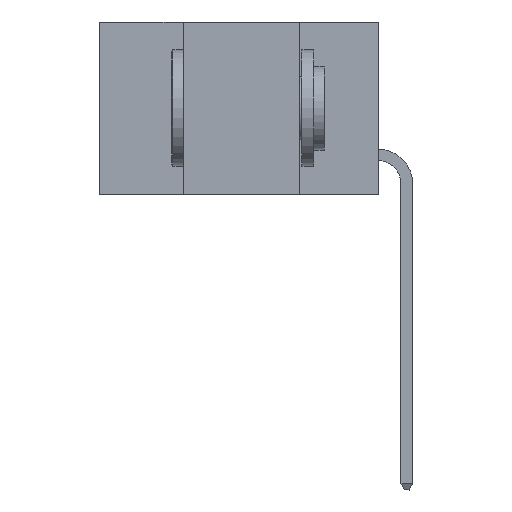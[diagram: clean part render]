
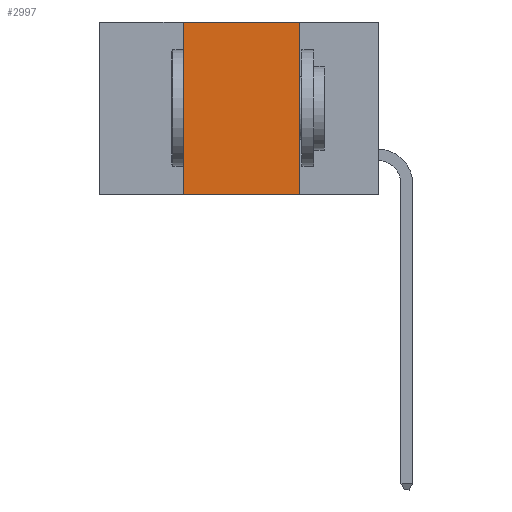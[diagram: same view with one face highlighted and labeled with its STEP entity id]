
A CAD part, left-side view. The second image highlights one B-rep face of the part: STEP entity #2997.
In plain terms, the highlighted planar face has unit normal (-1, 0, 0).
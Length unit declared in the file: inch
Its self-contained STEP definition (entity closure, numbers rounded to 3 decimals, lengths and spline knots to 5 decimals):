
#90 = ORIENTED_EDGE ( 'NONE', *, *, #4357, .F. ) ;
#1123 = LINE ( 'NONE', #12796, #13975 ) ;
#1261 = LINE ( 'NONE', #15414, #2188 ) ;
#2188 = VECTOR ( 'NONE', #5136, 39.37008 ) ;
#2242 = DIRECTION ( 'NONE',  ( 0., 0., 1. ) ) ;
#2484 = FACE_OUTER_BOUND ( 'NONE', #15917, .T. ) ;
#2997 = ADVANCED_FACE ( 'NONE', ( #2484 ), #16794, .F. ) ;
#3162 = CARTESIAN_POINT ( 'NONE',  ( 0., 0.17, 0. ) ) ;
#3624 = DIRECTION ( 'NONE',  ( 0., 0., -1. ) ) ;
#3863 = DIRECTION ( 'NONE',  ( 0., -1., 0. ) ) ;
#4176 = VERTEX_POINT ( 'NONE', #11252 ) ;
#4177 = EDGE_CURVE ( 'NONE', #8075, #9877, #13755, .T. ) ;
#4258 = EDGE_CURVE ( 'NONE', #10514, #4176, #1123, .T. ) ;
#4259 = VECTOR ( 'NONE', #3863, 39.37008 ) ;
#4357 = EDGE_CURVE ( 'NONE', #9877, #10514, #6378, .T. ) ;
#5136 = DIRECTION ( 'NONE',  ( 0., -1., 0. ) ) ;
#6006 = VECTOR ( 'NONE', #2242, 39.37008 ) ;
#6378 = LINE ( 'NONE', #11595, #4259 ) ;
#7236 = CARTESIAN_POINT ( 'NONE',  ( 0., 0.42, -0.37 ) ) ;
#8075 = VERTEX_POINT ( 'NONE', #9406 ) ;
#9406 = CARTESIAN_POINT ( 'NONE',  ( 0., 0.42, -0.37 ) ) ;
#9877 = VERTEX_POINT ( 'NONE', #12134 ) ;
#10135 = DIRECTION ( 'NONE',  ( 1., 0., 0. ) ) ;
#10378 = ORIENTED_EDGE ( 'NONE', *, *, #4177, .F. ) ;
#10514 = VERTEX_POINT ( 'NONE', #3162 ) ;
#11252 = CARTESIAN_POINT ( 'NONE',  ( 0., 0.17, -0.37 ) ) ;
#11595 = CARTESIAN_POINT ( 'NONE',  ( 0., 0.6, 0. ) ) ;
#11873 = ORIENTED_EDGE ( 'NONE', *, *, #4258, .F. ) ;
#11919 = AXIS2_PLACEMENT_3D ( 'NONE', #14090, #10135, #12709 ) ;
#12134 = CARTESIAN_POINT ( 'NONE',  ( 0., 0.42, 0. ) ) ;
#12396 = EDGE_CURVE ( 'NONE', #8075, #4176, #1261, .T. ) ;
#12709 = DIRECTION ( 'NONE',  ( 0., 0., -1. ) ) ;
#12796 = CARTESIAN_POINT ( 'NONE',  ( 0., 0.17, -0.37 ) ) ;
#13755 = LINE ( 'NONE', #7236, #6006 ) ;
#13975 = VECTOR ( 'NONE', #3624, 39.37008 ) ;
#14090 = CARTESIAN_POINT ( 'NONE',  ( 0., 0.6, 0. ) ) ;
#15414 = CARTESIAN_POINT ( 'NONE',  ( 0., 0.6, -0.37 ) ) ;
#15917 = EDGE_LOOP ( 'NONE', ( #11873, #90, #10378, #16892 ) ) ;
#16794 = PLANE ( 'NONE',  #11919 ) ;
#16892 = ORIENTED_EDGE ( 'NONE', *, *, #12396, .T. ) ;
